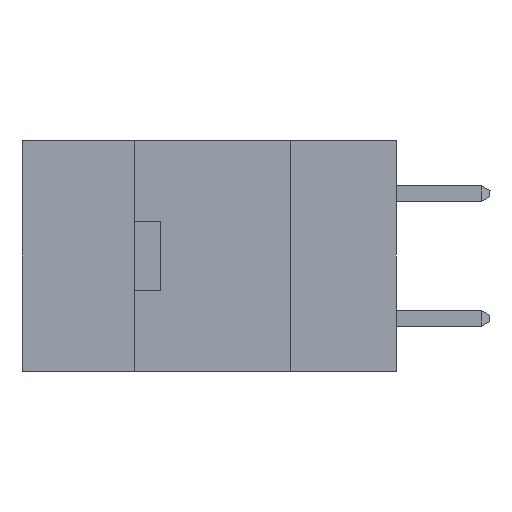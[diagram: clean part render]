
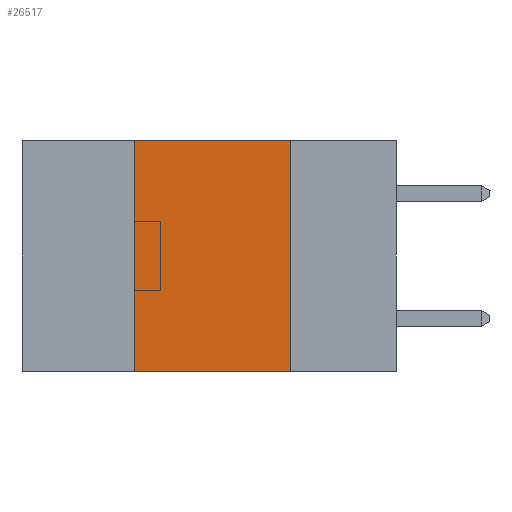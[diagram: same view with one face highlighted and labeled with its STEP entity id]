
A CAD part, left-side view. The second image highlights one B-rep face of the part: STEP entity #26517.
In plain terms, the highlighted planar face has unit normal (-1, 0, 0).
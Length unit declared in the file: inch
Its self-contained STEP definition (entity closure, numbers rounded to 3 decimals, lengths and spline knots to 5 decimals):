
#984 = LINE ( 'NONE', #20556, #11788 ) ;
#2450 = CARTESIAN_POINT ( 'NONE',  ( 0., 0.42, -0.37 ) ) ;
#2957 = VERTEX_POINT ( 'NONE', #14475 ) ;
#3187 = CARTESIAN_POINT ( 'NONE',  ( 0., 0.6, -0.37 ) ) ;
#3345 = PLANE ( 'NONE',  #8425 ) ;
#3831 = ORIENTED_EDGE ( 'NONE', *, *, #22333, .F. ) ;
#5113 = EDGE_CURVE ( 'NONE', #24224, #2957, #8796, .T. ) ;
#6403 = DIRECTION ( 'NONE',  ( 0., -1., 0. ) ) ;
#7671 = DIRECTION ( 'NONE',  ( 0., 0., -1. ) ) ;
#8425 = AXIS2_PLACEMENT_3D ( 'NONE', #18420, #20578, #7671 ) ;
#8634 = CARTESIAN_POINT ( 'NONE',  ( 0., 0.17, 0. ) ) ;
#8796 = LINE ( 'NONE', #2450, #19598 ) ;
#9891 = ORIENTED_EDGE ( 'NONE', *, *, #14114, .T. ) ;
#10165 = VERTEX_POINT ( 'NONE', #15702 ) ;
#10374 = LINE ( 'NONE', #21454, #21847 ) ;
#10923 = EDGE_LOOP ( 'NONE', ( #12588, #3831, #18013, #9891 ) ) ;
#11338 = VERTEX_POINT ( 'NONE', #8634 ) ;
#11788 = VECTOR ( 'NONE', #16247, 39.37008 ) ;
#12588 = ORIENTED_EDGE ( 'NONE', *, *, #21361, .F. ) ;
#14114 = EDGE_CURVE ( 'NONE', #24224, #10165, #15784, .T. ) ;
#14475 = CARTESIAN_POINT ( 'NONE',  ( 0., 0.42, 0. ) ) ;
#15702 = CARTESIAN_POINT ( 'NONE',  ( 0., 0.17, -0.37 ) ) ;
#15784 = LINE ( 'NONE', #3187, #25812 ) ;
#16247 = DIRECTION ( 'NONE',  ( 0., 0., -1. ) ) ;
#17481 = CARTESIAN_POINT ( 'NONE',  ( 0., 0.42, -0.37 ) ) ;
#17512 = DIRECTION ( 'NONE',  ( 0., 0., 1. ) ) ;
#18013 = ORIENTED_EDGE ( 'NONE', *, *, #5113, .F. ) ;
#18420 = CARTESIAN_POINT ( 'NONE',  ( 0., 0.6, 0. ) ) ;
#19598 = VECTOR ( 'NONE', #17512, 39.37008 ) ;
#20556 = CARTESIAN_POINT ( 'NONE',  ( 0., 0.17, -0.37 ) ) ;
#20578 = DIRECTION ( 'NONE',  ( 1., 0., 0. ) ) ;
#21361 = EDGE_CURVE ( 'NONE', #11338, #10165, #984, .T. ) ;
#21454 = CARTESIAN_POINT ( 'NONE',  ( 0., 0.6, 0. ) ) ;
#21847 = VECTOR ( 'NONE', #6403, 39.37008 ) ;
#22333 = EDGE_CURVE ( 'NONE', #2957, #11338, #10374, .T. ) ;
#24224 = VERTEX_POINT ( 'NONE', #17481 ) ;
#25812 = VECTOR ( 'NONE', #26842, 39.37008 ) ;
#26517 = ADVANCED_FACE ( 'NONE', ( #27592 ), #3345, .F. ) ;
#26842 = DIRECTION ( 'NONE',  ( 0., -1., 0. ) ) ;
#27592 = FACE_OUTER_BOUND ( 'NONE', #10923, .T. ) ;
